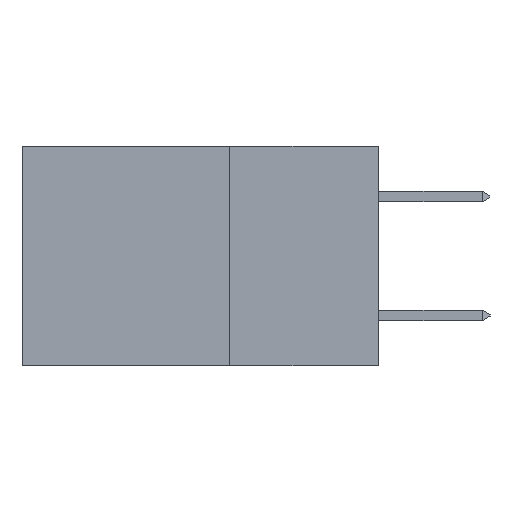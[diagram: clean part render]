
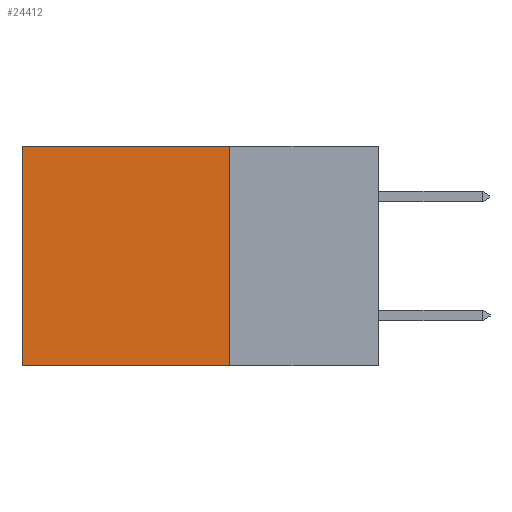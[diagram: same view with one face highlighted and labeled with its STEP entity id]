
A CAD part, left-side view. The second image highlights one B-rep face of the part: STEP entity #24412.
In plain terms, the highlighted planar face has unit normal (-1, 0, 0).
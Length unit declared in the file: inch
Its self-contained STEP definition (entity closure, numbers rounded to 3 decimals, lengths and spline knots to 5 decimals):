
#14 = LINE ( 'NONE', #22530, #16306 ) ;
#971 = VERTEX_POINT ( 'NONE', #18650 ) ;
#3562 = EDGE_CURVE ( 'NONE', #9453, #15190, #12189, .T. ) ;
#3879 = EDGE_CURVE ( 'NONE', #971, #9453, #16175, .T. ) ;
#3983 = DIRECTION ( 'NONE',  ( 0., 0., -1. ) ) ;
#4912 = DIRECTION ( 'NONE',  ( 0., 0., -1. ) ) ;
#5745 = EDGE_CURVE ( 'NONE', #11391, #15190, #14408, .T. ) ;
#5789 = FACE_OUTER_BOUND ( 'NONE', #18387, .T. ) ;
#6544 = VECTOR ( 'NONE', #13686, 39.37008 ) ;
#7279 = CARTESIAN_POINT ( 'NONE',  ( 0.2615, 0.25, -0.37 ) ) ;
#8498 = ORIENTED_EDGE ( 'NONE', *, *, #3562, .F. ) ;
#9453 = VERTEX_POINT ( 'NONE', #7279 ) ;
#9827 = ORIENTED_EDGE ( 'NONE', *, *, #5745, .T. ) ;
#11197 = CARTESIAN_POINT ( 'NONE',  ( 0.2615, 0.25, -0.37 ) ) ;
#11391 = VERTEX_POINT ( 'NONE', #12075 ) ;
#12075 = CARTESIAN_POINT ( 'NONE',  ( 0.2615, 0.6, 0. ) ) ;
#12189 = LINE ( 'NONE', #20944, #6544 ) ;
#12746 = EDGE_CURVE ( 'NONE', #971, #11391, #14, .T. ) ;
#12926 = ORIENTED_EDGE ( 'NONE', *, *, #3879, .F. ) ;
#13371 = CARTESIAN_POINT ( 'NONE',  ( 0.2615, 0.6, -0.37 ) ) ;
#13686 = DIRECTION ( 'NONE',  ( 0., 1., 0. ) ) ;
#14408 = LINE ( 'NONE', #13371, #24909 ) ;
#14606 = PLANE ( 'NONE',  #27110 ) ;
#14853 = VECTOR ( 'NONE', #25947, 39.37008 ) ;
#15190 = VERTEX_POINT ( 'NONE', #18070 ) ;
#16175 = LINE ( 'NONE', #11197, #14853 ) ;
#16306 = VECTOR ( 'NONE', #20317, 39.37008 ) ;
#16701 = DIRECTION ( 'NONE',  ( 1., 0., 0. ) ) ;
#18070 = CARTESIAN_POINT ( 'NONE',  ( 0.2615, 0.6, -0.37 ) ) ;
#18387 = EDGE_LOOP ( 'NONE', ( #9827, #8498, #12926, #23697 ) ) ;
#18650 = CARTESIAN_POINT ( 'NONE',  ( 0.2615, 0.25, 0. ) ) ;
#20317 = DIRECTION ( 'NONE',  ( 0., 1., 0. ) ) ;
#20841 = CARTESIAN_POINT ( 'NONE',  ( 0.2615, 0.25, -0.37 ) ) ;
#20944 = CARTESIAN_POINT ( 'NONE',  ( 0.2615, 0.25, -0.37 ) ) ;
#22530 = CARTESIAN_POINT ( 'NONE',  ( 0.2615, 0.25, 0. ) ) ;
#23697 = ORIENTED_EDGE ( 'NONE', *, *, #12746, .T. ) ;
#24412 = ADVANCED_FACE ( 'NONE', ( #5789 ), #14606, .F. ) ;
#24909 = VECTOR ( 'NONE', #4912, 39.37008 ) ;
#25947 = DIRECTION ( 'NONE',  ( 0., 0., -1. ) ) ;
#27110 = AXIS2_PLACEMENT_3D ( 'NONE', #20841, #16701, #3983 ) ;
